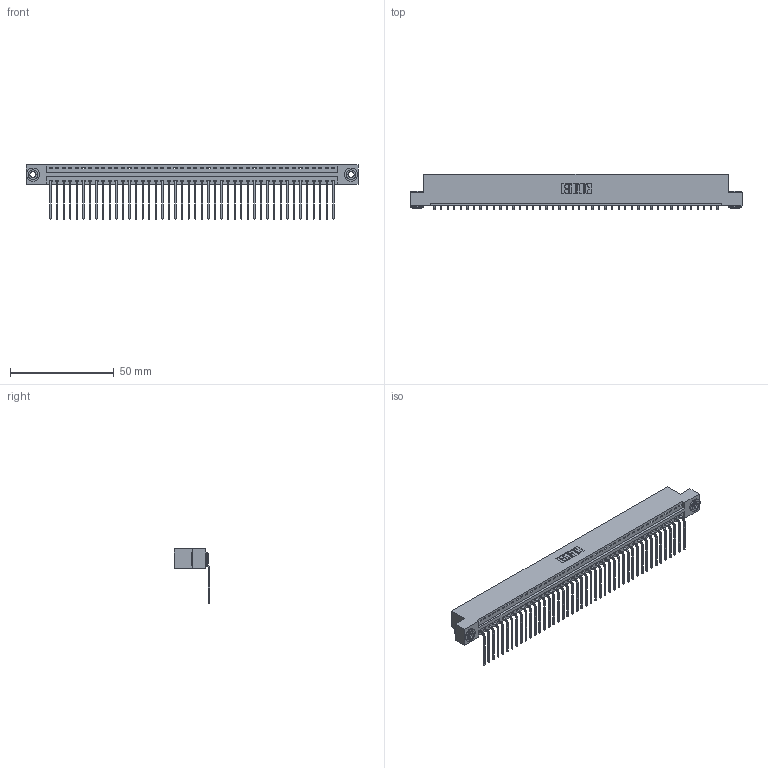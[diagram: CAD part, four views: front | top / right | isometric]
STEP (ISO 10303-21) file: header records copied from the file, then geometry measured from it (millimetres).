
FILE_DESCRIPTION (( 'STEP AP203' ), '1' );
FILE_NAME ('346-044-559-103.STEP', '2022-05-09T17:42:22', ( '' ), ( '' ), 'SwSTEP 2.0', 'SolidWorks 2020', '' );
FILE_SCHEMA (( 'CONFIG_CONTROL_DESIGN' ));
Length unit declared in the file: inch
Products named in the file (4): 346-044-559-103; 345-250-002_345-250-002-102; 346 Part_Flush Mounting Lugs - 0.156 Dia-TH; 345-292-001_558 559 Tail - 1
Assembly tree (47 placements, depth 2):
  346-044-559-103
    346 Part_Flush Mounting Lugs - 0.156 Dia-TH
    345-292-001_558 559 Tail - 1  x44
    345-250-002_345-250-002-102  x2
Bounding box: 160.27 x 17.08 x 26.16 mm (x, y, z)
Volume: 15503.4 mm3; surface area: 20524.9 mm2
Topology: 47 solids, 47 shells, 2814 faces, 8449 edges, 5570 vertices
Faces by surface type: plane 1948, cylinder 858, cone 8
Entity records: 28188 total; most frequent: CARTESIAN_POINT 4813, ORIENTED_EDGE 4782, DIRECTION 4273, EDGE_CURVE 2391, LINE 2059, VECTOR 2059, VERTEX_POINT 1590, AXIS2_PLACEMENT_3D 1107
